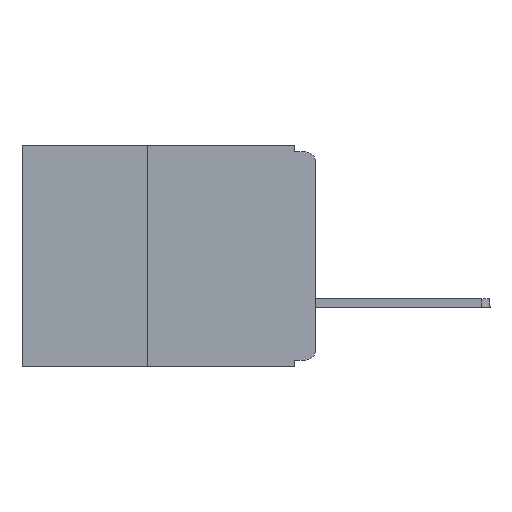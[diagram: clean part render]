
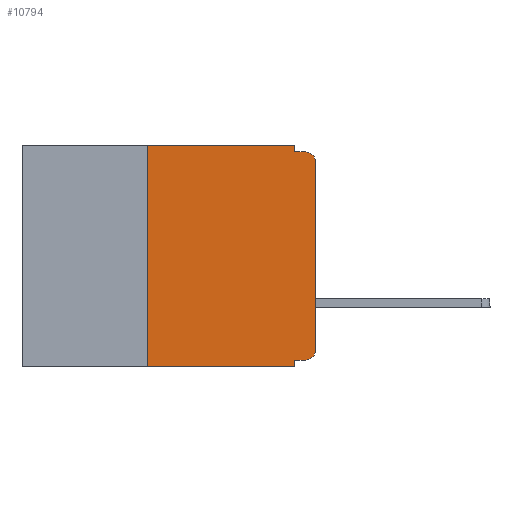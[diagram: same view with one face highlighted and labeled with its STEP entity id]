
A CAD part, left-side view. The second image highlights one B-rep face of the part: STEP entity #10794.
In plain terms, the highlighted planar face has unit normal (-1, 0, 0).
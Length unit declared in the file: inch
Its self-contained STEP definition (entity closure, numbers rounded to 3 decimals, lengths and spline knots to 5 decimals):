
#120 = VERTEX_POINT ( 'NONE', #9244 ) ;
#504 = VECTOR ( 'NONE', #2933, 39.37008 ) ;
#618 = EDGE_CURVE ( 'NONE', #5815, #22046, #9380, .T. ) ;
#772 = CARTESIAN_POINT ( 'NONE',  ( 0., 0., -0.305 ) ) ;
#964 = ORIENTED_EDGE ( 'NONE', *, *, #23250, .F. ) ;
#2009 = EDGE_CURVE ( 'NONE', #14999, #11663, #19018, .T. ) ;
#2185 = DIRECTION ( 'NONE',  ( -1., 0., 0. ) ) ;
#2596 = DIRECTION ( 'NONE',  ( 0., 0., 1. ) ) ;
#2639 = CARTESIAN_POINT ( 'NONE',  ( 0., 0.031, -0.33 ) ) ;
#2933 = DIRECTION ( 'NONE',  ( 0., 0., -1. ) ) ;
#3093 = DIRECTION ( 'NONE',  ( 0., 0., -1. ) ) ;
#3248 = EDGE_CURVE ( 'NONE', #11911, #16192, #20948, .T. ) ;
#4009 = DIRECTION ( 'NONE',  ( -1., 0., 0. ) ) ;
#4344 = CARTESIAN_POINT ( 'NONE',  ( 0., 0.015, -0.32 ) ) ;
#4565 = CARTESIAN_POINT ( 'NONE',  ( 0., 0., -0.32 ) ) ;
#4748 = CARTESIAN_POINT ( 'NONE',  ( 0., 0.437, -0.33 ) ) ;
#5354 = FACE_OUTER_BOUND ( 'NONE', #8745, .T. ) ;
#5488 = CIRCLE ( 'NONE', #8240, 0.015 ) ;
#5527 = VERTEX_POINT ( 'NONE', #4344 ) ;
#5815 = VERTEX_POINT ( 'NONE', #17967 ) ;
#5851 = VECTOR ( 'NONE', #19138, 39.37008 ) ;
#6003 = LINE ( 'NONE', #4748, #10279 ) ;
#7118 = AXIS2_PLACEMENT_3D ( 'NONE', #8538, #14046, #3093 ) ;
#7630 = AXIS2_PLACEMENT_3D ( 'NONE', #14966, #4009, #16776 ) ;
#7965 = VERTEX_POINT ( 'NONE', #2639 ) ;
#8240 = AXIS2_PLACEMENT_3D ( 'NONE', #13110, #2185, #14959 ) ;
#8538 = CARTESIAN_POINT ( 'NONE',  ( 0., 0.437, 0. ) ) ;
#8745 = EDGE_LOOP ( 'NONE', ( #15055, #11319, #11580, #23068, #964, #20714, #10716, #21710, #22816, #20909 ) ) ;
#9073 = CARTESIAN_POINT ( 'NONE',  ( 0., 0.25, 0. ) ) ;
#9244 = CARTESIAN_POINT ( 'NONE',  ( 0., 0.015, -0.01 ) ) ;
#9380 = LINE ( 'NONE', #19399, #22685 ) ;
#9922 = EDGE_CURVE ( 'NONE', #22046, #120, #13975, .T. ) ;
#10279 = VECTOR ( 'NONE', #15678, 39.37008 ) ;
#10716 = ORIENTED_EDGE ( 'NONE', *, *, #18512, .T. ) ;
#10770 = EDGE_CURVE ( 'NONE', #11380, #7965, #19889, .T. ) ;
#10794 = ADVANCED_FACE ( 'NONE', ( #5354 ), #17602, .F. ) ;
#10892 = DIRECTION ( 'NONE',  ( 0., 0., 1. ) ) ;
#11171 = CARTESIAN_POINT ( 'NONE',  ( 0., 0.25, -0.33 ) ) ;
#11319 = ORIENTED_EDGE ( 'NONE', *, *, #20787, .T. ) ;
#11380 = VERTEX_POINT ( 'NONE', #11545 ) ;
#11545 = CARTESIAN_POINT ( 'NONE',  ( 0., 0.031, -0.32 ) ) ;
#11580 = ORIENTED_EDGE ( 'NONE', *, *, #9922, .F. ) ;
#11657 = CARTESIAN_POINT ( 'NONE',  ( 0., 0., -0.01 ) ) ;
#11663 = VERTEX_POINT ( 'NONE', #9073 ) ;
#11911 = VERTEX_POINT ( 'NONE', #772 ) ;
#13110 = CARTESIAN_POINT ( 'NONE',  ( 0., 0.015, -0.025 ) ) ;
#13615 = VECTOR ( 'NONE', #10892, 39.37008 ) ;
#13975 = LINE ( 'NONE', #11657, #18221 ) ;
#14046 = DIRECTION ( 'NONE',  ( 1., 0., 0. ) ) ;
#14219 = CARTESIAN_POINT ( 'NONE',  ( 0., 0., -0.025 ) ) ;
#14959 = DIRECTION ( 'NONE',  ( 0., 0., -1. ) ) ;
#14966 = CARTESIAN_POINT ( 'NONE',  ( 0., 0.015, -0.305 ) ) ;
#14999 = VERTEX_POINT ( 'NONE', #16314 ) ;
#15055 = ORIENTED_EDGE ( 'NONE', *, *, #3248, .T. ) ;
#15147 = EDGE_CURVE ( 'NONE', #5527, #11911, #18441, .T. ) ;
#15362 = CARTESIAN_POINT ( 'NONE',  ( 0., 0., 0. ) ) ;
#15478 = VECTOR ( 'NONE', #17739, 39.37008 ) ;
#15678 = DIRECTION ( 'NONE',  ( 0., -1., 0. ) ) ;
#15926 = CARTESIAN_POINT ( 'NONE',  ( 0., 0.437, 0. ) ) ;
#16192 = VERTEX_POINT ( 'NONE', #14219 ) ;
#16314 = CARTESIAN_POINT ( 'NONE',  ( 0., 0.25, -0.33 ) ) ;
#16776 = DIRECTION ( 'NONE',  ( 0., 0., -1. ) ) ;
#16782 = DIRECTION ( 'NONE',  ( 0., 0., -1. ) ) ;
#17285 = VECTOR ( 'NONE', #2596, 39.37008 ) ;
#17602 = PLANE ( 'NONE',  #7118 ) ;
#17739 = DIRECTION ( 'NONE',  ( 0., -1., 0. ) ) ;
#17967 = CARTESIAN_POINT ( 'NONE',  ( 0., 0.031, 0. ) ) ;
#18221 = VECTOR ( 'NONE', #18912, 39.37008 ) ;
#18441 = CIRCLE ( 'NONE', #7630, 0.015 ) ;
#18512 = EDGE_CURVE ( 'NONE', #14999, #7965, #6003, .T. ) ;
#18912 = DIRECTION ( 'NONE',  ( 0., -1., 0. ) ) ;
#19018 = LINE ( 'NONE', #11171, #13615 ) ;
#19138 = DIRECTION ( 'NONE',  ( 0., 1., 0. ) ) ;
#19302 = CARTESIAN_POINT ( 'NONE',  ( 0., 0.031, -0.01 ) ) ;
#19399 = CARTESIAN_POINT ( 'NONE',  ( 0., 0.031, 0. ) ) ;
#19889 = LINE ( 'NONE', #21143, #504 ) ;
#20287 = LINE ( 'NONE', #15926, #15478 ) ;
#20354 = LINE ( 'NONE', #4565, #5851 ) ;
#20714 = ORIENTED_EDGE ( 'NONE', *, *, #2009, .F. ) ;
#20787 = EDGE_CURVE ( 'NONE', #16192, #120, #5488, .T. ) ;
#20909 = ORIENTED_EDGE ( 'NONE', *, *, #15147, .T. ) ;
#20948 = LINE ( 'NONE', #15362, #17285 ) ;
#21143 = CARTESIAN_POINT ( 'NONE',  ( 0., 0.031, -0.33 ) ) ;
#21710 = ORIENTED_EDGE ( 'NONE', *, *, #10770, .F. ) ;
#22004 = EDGE_CURVE ( 'NONE', #5527, #11380, #20354, .T. ) ;
#22046 = VERTEX_POINT ( 'NONE', #19302 ) ;
#22685 = VECTOR ( 'NONE', #16782, 39.37008 ) ;
#22816 = ORIENTED_EDGE ( 'NONE', *, *, #22004, .F. ) ;
#23068 = ORIENTED_EDGE ( 'NONE', *, *, #618, .F. ) ;
#23250 = EDGE_CURVE ( 'NONE', #11663, #5815, #20287, .T. ) ;
